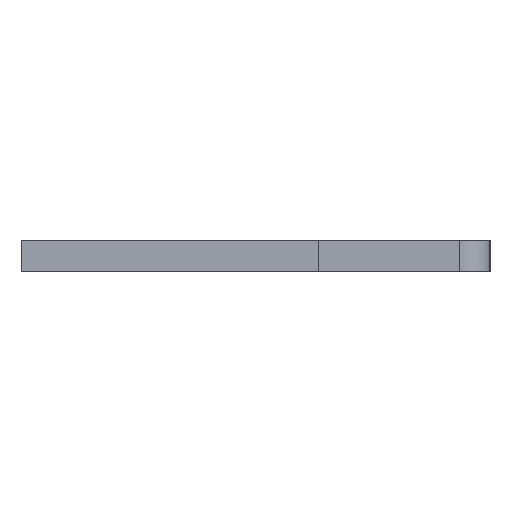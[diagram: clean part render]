
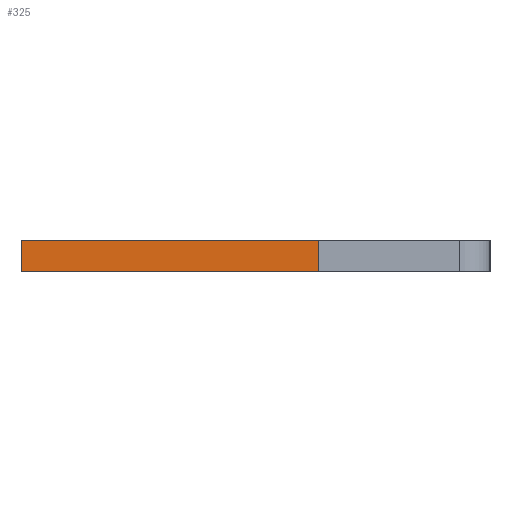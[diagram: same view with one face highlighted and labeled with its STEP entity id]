
A CAD part, left-side view. The second image highlights one B-rep face of the part: STEP entity #325.
In plain terms, the highlighted face is planar.
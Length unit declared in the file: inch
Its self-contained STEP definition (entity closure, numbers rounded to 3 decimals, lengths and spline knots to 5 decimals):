
#24 = CARTESIAN_POINT ( 'NONE',  ( -0.01, 0.15, -0.04 ) ) ;
#46 = LINE ( 'NONE', #1030, #887 ) ;
#58 = DIRECTION ( 'NONE',  ( -1., 0., 0. ) ) ;
#122 = VECTOR ( 'NONE', #395, 39.37008 ) ;
#143 = VERTEX_POINT ( 'NONE', #24 ) ;
#188 = VECTOR ( 'NONE', #688, 39.37008 ) ;
#209 = CARTESIAN_POINT ( 'NONE',  ( 0.01, 0.15, -0.04 ) ) ;
#213 = FACE_OUTER_BOUND ( 'NONE', #910, .T. ) ;
#270 = DIRECTION ( 'NONE',  ( 0., 0., 1. ) ) ;
#325 = ADVANCED_FACE ( 'NONE', ( #213 ), #447, .F. ) ;
#327 = VERTEX_POINT ( 'NONE', #347 ) ;
#347 = CARTESIAN_POINT ( 'NONE',  ( -0.01, -0.04, -0.04 ) ) ;
#395 = DIRECTION ( 'NONE',  ( 0., 1., 0. ) ) ;
#405 = LINE ( 'NONE', #442, #188 ) ;
#424 = EDGE_CURVE ( 'NONE', #327, #143, #405, .T. ) ;
#442 = CARTESIAN_POINT ( 'NONE',  ( -0.01, 0.15, -0.04 ) ) ;
#447 = PLANE ( 'NONE',  #475 ) ;
#466 = CARTESIAN_POINT ( 'NONE',  ( 0.01, 0.15, -0.04 ) ) ;
#475 = AXIS2_PLACEMENT_3D ( 'NONE', #837, #270, #1009 ) ;
#593 = VERTEX_POINT ( 'NONE', #864 ) ;
#610 = LINE ( 'NONE', #209, #122 ) ;
#653 = DIRECTION ( 'NONE',  ( -1., 0., 0. ) ) ;
#687 = EDGE_CURVE ( 'NONE', #843, #143, #46, .T. ) ;
#688 = DIRECTION ( 'NONE',  ( 0., 1., 0. ) ) ;
#700 = ORIENTED_EDGE ( 'NONE', *, *, #759, .F. ) ;
#759 = EDGE_CURVE ( 'NONE', #593, #843, #610, .T. ) ;
#837 = CARTESIAN_POINT ( 'NONE',  ( 0.01, 0.15, -0.04 ) ) ;
#843 = VERTEX_POINT ( 'NONE', #466 ) ;
#854 = ORIENTED_EDGE ( 'NONE', *, *, #687, .F. ) ;
#864 = CARTESIAN_POINT ( 'NONE',  ( 0.01, -0.04, -0.04 ) ) ;
#880 = ORIENTED_EDGE ( 'NONE', *, *, #424, .T. ) ;
#887 = VECTOR ( 'NONE', #58, 39.37008 ) ;
#892 = LINE ( 'NONE', #894, #952 ) ;
#894 = CARTESIAN_POINT ( 'NONE',  ( 0.01, -0.04, -0.04 ) ) ;
#910 = EDGE_LOOP ( 'NONE', ( #880, #854, #700, #1008 ) ) ;
#952 = VECTOR ( 'NONE', #653, 39.37008 ) ;
#999 = EDGE_CURVE ( 'NONE', #593, #327, #892, .T. ) ;
#1008 = ORIENTED_EDGE ( 'NONE', *, *, #999, .T. ) ;
#1009 = DIRECTION ( 'NONE',  ( 1., 0., 0. ) ) ;
#1030 = CARTESIAN_POINT ( 'NONE',  ( 0.01, 0.15, -0.04 ) ) ;
